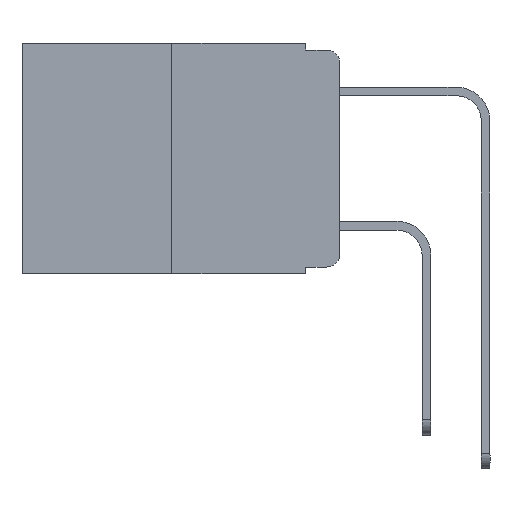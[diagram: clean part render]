
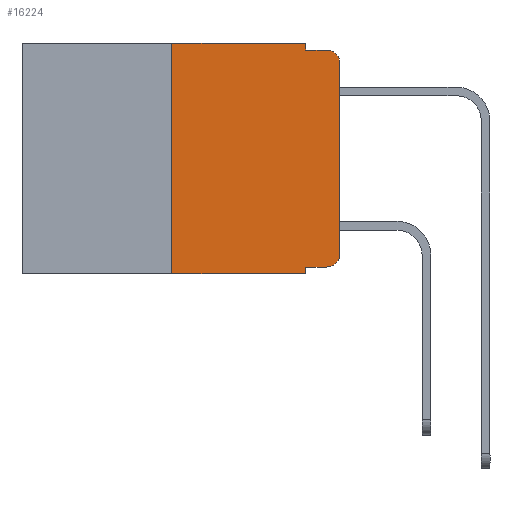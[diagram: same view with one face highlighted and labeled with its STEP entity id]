
A CAD part, left-side view. The second image highlights one B-rep face of the part: STEP entity #16224.
In plain terms, the highlighted planar face has unit normal (-1, 0, 0).
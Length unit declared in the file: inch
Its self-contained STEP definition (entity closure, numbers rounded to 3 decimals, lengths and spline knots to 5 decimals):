
#253 = LINE ( 'NONE', #10769, #18670 ) ;
#259 = VERTEX_POINT ( 'NONE', #5102 ) ;
#450 = VECTOR ( 'NONE', #3893, 39.37008 ) ;
#758 = VECTOR ( 'NONE', #17384, 39.37008 ) ;
#832 = LINE ( 'NONE', #2537, #20068 ) ;
#1003 = CARTESIAN_POINT ( 'NONE',  ( 0., 0.051, -0.01 ) ) ;
#1019 = CARTESIAN_POINT ( 'NONE',  ( 0., 0., -0.03 ) ) ;
#1690 = CARTESIAN_POINT ( 'NONE',  ( 0., 0.02, -0.03 ) ) ;
#1881 = DIRECTION ( 'NONE',  ( 1., 0., 0. ) ) ;
#2300 = LINE ( 'NONE', #17940, #450 ) ;
#2537 = CARTESIAN_POINT ( 'NONE',  ( 0., 0.051, -0.333 ) ) ;
#2797 = VERTEX_POINT ( 'NONE', #1019 ) ;
#2968 = EDGE_CURVE ( 'NONE', #2797, #3064, #11202, .T. ) ;
#3023 = AXIS2_PLACEMENT_3D ( 'NONE', #1690, #11784, #10066 ) ;
#3064 = VERTEX_POINT ( 'NONE', #5752 ) ;
#3130 = ORIENTED_EDGE ( 'NONE', *, *, #5975, .T. ) ;
#3432 = CIRCLE ( 'NONE', #7073, 0.02 ) ;
#3587 = EDGE_CURVE ( 'NONE', #4098, #9086, #10470, .T. ) ;
#3713 = CARTESIAN_POINT ( 'NONE',  ( 0., 0.25, 0. ) ) ;
#3777 = VERTEX_POINT ( 'NONE', #6737 ) ;
#3862 = CARTESIAN_POINT ( 'NONE',  ( 0., 0., 0. ) ) ;
#3893 = DIRECTION ( 'NONE',  ( 0., 0., -1. ) ) ;
#4084 = DIRECTION ( 'NONE',  ( 0., -1., 0. ) ) ;
#4098 = VERTEX_POINT ( 'NONE', #21225 ) ;
#4125 = CARTESIAN_POINT ( 'NONE',  ( 0., 0.051, -0.343 ) ) ;
#4874 = VECTOR ( 'NONE', #4084, 39.37008 ) ;
#5102 = CARTESIAN_POINT ( 'NONE',  ( 0., 0., -0.313 ) ) ;
#5457 = ORIENTED_EDGE ( 'NONE', *, *, #2968, .T. ) ;
#5615 = CARTESIAN_POINT ( 'NONE',  ( 0., 0.25, 0. ) ) ;
#5752 = CARTESIAN_POINT ( 'NONE',  ( 0., 0.02, -0.01 ) ) ;
#5975 = EDGE_CURVE ( 'NONE', #259, #2797, #8957, .T. ) ;
#6006 = CARTESIAN_POINT ( 'NONE',  ( 0., 0.02, -0.313 ) ) ;
#6058 = ORIENTED_EDGE ( 'NONE', *, *, #7813, .F. ) ;
#6292 = VECTOR ( 'NONE', #12922, 39.37008 ) ;
#6737 = CARTESIAN_POINT ( 'NONE',  ( 0., 0.051, 0. ) ) ;
#7073 = AXIS2_PLACEMENT_3D ( 'NONE', #6006, #19815, #13265 ) ;
#7226 = ORIENTED_EDGE ( 'NONE', *, *, #15375, .F. ) ;
#7449 = FACE_OUTER_BOUND ( 'NONE', #18723, .T. ) ;
#7813 = EDGE_CURVE ( 'NONE', #3777, #16500, #9722, .T. ) ;
#7979 = DIRECTION ( 'NONE',  ( 0., -1., 0. ) ) ;
#8338 = ORIENTED_EDGE ( 'NONE', *, *, #18527, .F. ) ;
#8957 = LINE ( 'NONE', #3862, #12777 ) ;
#9086 = VERTEX_POINT ( 'NONE', #3713 ) ;
#9348 = CARTESIAN_POINT ( 'NONE',  ( 0., 0.02, -0.333 ) ) ;
#9375 = DIRECTION ( 'NONE',  ( 0., 0., -1. ) ) ;
#9712 = ORIENTED_EDGE ( 'NONE', *, *, #3587, .F. ) ;
#9722 = LINE ( 'NONE', #16639, #9948 ) ;
#9948 = VECTOR ( 'NONE', #9375, 39.37008 ) ;
#10066 = DIRECTION ( 'NONE',  ( 0., 0., -1. ) ) ;
#10390 = DIRECTION ( 'NONE',  ( 0., 0., -1. ) ) ;
#10470 = LINE ( 'NONE', #5615, #758 ) ;
#10658 = DIRECTION ( 'NONE',  ( 0., -1., 0. ) ) ;
#10769 = CARTESIAN_POINT ( 'NONE',  ( 0., 0.473, 0. ) ) ;
#11202 = CIRCLE ( 'NONE', #3023, 0.02 ) ;
#11784 = DIRECTION ( 'NONE',  ( -1., 0., 0. ) ) ;
#12104 = PLANE ( 'NONE',  #20694 ) ;
#12543 = ORIENTED_EDGE ( 'NONE', *, *, #12741, .T. ) ;
#12741 = EDGE_CURVE ( 'NONE', #18869, #13255, #832, .T. ) ;
#12777 = VECTOR ( 'NONE', #17782, 39.37008 ) ;
#12922 = DIRECTION ( 'NONE',  ( 0., -1., 0. ) ) ;
#12995 = ORIENTED_EDGE ( 'NONE', *, *, #14716, .T. ) ;
#13255 = VERTEX_POINT ( 'NONE', #9348 ) ;
#13265 = DIRECTION ( 'NONE',  ( 0., 0., -1. ) ) ;
#14137 = EDGE_CURVE ( 'NONE', #4098, #16710, #14172, .T. ) ;
#14172 = LINE ( 'NONE', #17919, #4874 ) ;
#14716 = EDGE_CURVE ( 'NONE', #13255, #259, #3432, .T. ) ;
#14823 = LINE ( 'NONE', #1003, #6292 ) ;
#15375 = EDGE_CURVE ( 'NONE', #9086, #3777, #253, .T. ) ;
#15469 = ORIENTED_EDGE ( 'NONE', *, *, #19508, .F. ) ;
#15868 = CARTESIAN_POINT ( 'NONE',  ( 0., 0.051, -0.333 ) ) ;
#16224 = ADVANCED_FACE ( 'NONE', ( #7449 ), #12104, .F. ) ;
#16500 = VERTEX_POINT ( 'NONE', #20570 ) ;
#16639 = CARTESIAN_POINT ( 'NONE',  ( 0., 0.051, 0. ) ) ;
#16710 = VERTEX_POINT ( 'NONE', #4125 ) ;
#17384 = DIRECTION ( 'NONE',  ( 0., 0., 1. ) ) ;
#17782 = DIRECTION ( 'NONE',  ( 0., 0., 1. ) ) ;
#17919 = CARTESIAN_POINT ( 'NONE',  ( 0., 0.473, -0.343 ) ) ;
#17940 = CARTESIAN_POINT ( 'NONE',  ( 0., 0.051, 0. ) ) ;
#18234 = ORIENTED_EDGE ( 'NONE', *, *, #14137, .T. ) ;
#18527 = EDGE_CURVE ( 'NONE', #18869, #16710, #2300, .T. ) ;
#18670 = VECTOR ( 'NONE', #10658, 39.37008 ) ;
#18723 = EDGE_LOOP ( 'NONE', ( #3130, #5457, #15469, #6058, #7226, #9712, #18234, #8338, #12543, #12995 ) ) ;
#18869 = VERTEX_POINT ( 'NONE', #15868 ) ;
#19015 = CARTESIAN_POINT ( 'NONE',  ( 0., 0.473, 0. ) ) ;
#19508 = EDGE_CURVE ( 'NONE', #16500, #3064, #14823, .T. ) ;
#19815 = DIRECTION ( 'NONE',  ( -1., 0., 0. ) ) ;
#20068 = VECTOR ( 'NONE', #7979, 39.37008 ) ;
#20570 = CARTESIAN_POINT ( 'NONE',  ( 0., 0.051, -0.01 ) ) ;
#20694 = AXIS2_PLACEMENT_3D ( 'NONE', #19015, #1881, #10390 ) ;
#21225 = CARTESIAN_POINT ( 'NONE',  ( 0., 0.25, -0.343 ) ) ;
